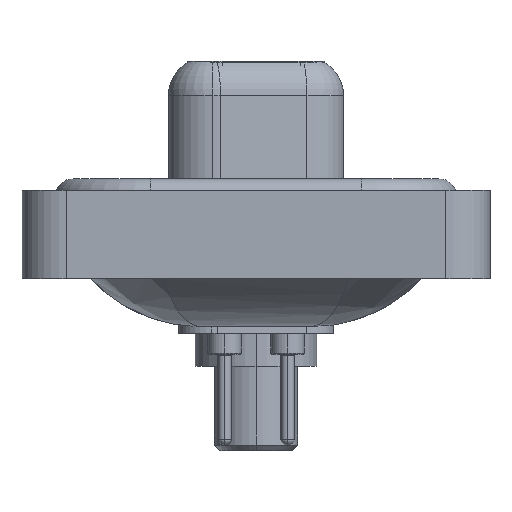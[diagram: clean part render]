
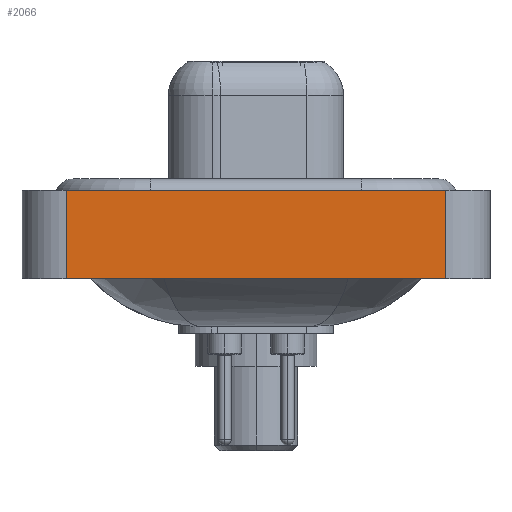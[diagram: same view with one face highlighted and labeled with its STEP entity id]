
A CAD part, left-side view. The second image highlights one B-rep face of the part: STEP entity #2066.
In plain terms, the highlighted planar face has unit normal (-1, 0, 0).
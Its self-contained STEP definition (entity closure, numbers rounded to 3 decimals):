
#321 = DIRECTION ( 'NONE',  ( 0., -1., 0. ) ) ;
#752 = LINE ( 'NONE', #3815, #19034 ) ;
#1023 = CARTESIAN_POINT ( 'NONE',  ( -7.25, -8.55, -3.6 ) ) ;
#1739 = ORIENTED_EDGE ( 'NONE', *, *, #3732, .F. ) ;
#2066 = ADVANCED_FACE ( 'NONE', ( #14321 ), #18576, .T. ) ;
#2612 = VECTOR ( 'NONE', #8266, 1000. ) ;
#2680 = VERTEX_POINT ( 'NONE', #13771 ) ;
#2856 = DIRECTION ( 'NONE',  ( 0., 0., 1. ) ) ;
#3732 = EDGE_CURVE ( 'NONE', #5099, #2680, #752, .T. ) ;
#3815 = CARTESIAN_POINT ( 'NONE',  ( -7.25, 8.55, -3.6 ) ) ;
#4140 = LINE ( 'NONE', #16198, #8108 ) ;
#4778 = VECTOR ( 'NONE', #321, 1000. ) ;
#4995 = ORIENTED_EDGE ( 'NONE', *, *, #15892, .T. ) ;
#5099 = VERTEX_POINT ( 'NONE', #9161 ) ;
#5203 = LINE ( 'NONE', #15603, #2612 ) ;
#6638 = EDGE_CURVE ( 'NONE', #2680, #16974, #8024, .T. ) ;
#6761 = DIRECTION ( 'NONE',  ( 0., 0., 1. ) ) ;
#6812 = ORIENTED_EDGE ( 'NONE', *, *, #9829, .T. ) ;
#8024 = LINE ( 'NONE', #17024, #4778 ) ;
#8108 = VECTOR ( 'NONE', #2856, 1000. ) ;
#8266 = DIRECTION ( 'NONE',  ( 0., -1., 0. ) ) ;
#9161 = CARTESIAN_POINT ( 'NONE',  ( -7.25, 8.55, -3.6 ) ) ;
#9829 = EDGE_CURVE ( 'NONE', #5099, #14279, #5203, .T. ) ;
#12650 = CARTESIAN_POINT ( 'NONE',  ( -7.25, -8.55, -3.6 ) ) ;
#13771 = CARTESIAN_POINT ( 'NONE',  ( -7.25, 8.55, 0.4 ) ) ;
#13804 = AXIS2_PLACEMENT_3D ( 'NONE', #12650, #14416, #18670 ) ;
#14279 = VERTEX_POINT ( 'NONE', #1023 ) ;
#14321 = FACE_OUTER_BOUND ( 'NONE', #16238, .T. ) ;
#14416 = DIRECTION ( 'NONE',  ( -1., 0., 0. ) ) ;
#15603 = CARTESIAN_POINT ( 'NONE',  ( -7.25, -8.55, -3.6 ) ) ;
#15892 = EDGE_CURVE ( 'NONE', #14279, #16974, #4140, .T. ) ;
#16198 = CARTESIAN_POINT ( 'NONE',  ( -7.25, -8.55, -3.6 ) ) ;
#16238 = EDGE_LOOP ( 'NONE', ( #4995, #18904, #1739, #6812 ) ) ;
#16623 = CARTESIAN_POINT ( 'NONE',  ( -7.25, -8.55, 0.4 ) ) ;
#16974 = VERTEX_POINT ( 'NONE', #16623 ) ;
#17024 = CARTESIAN_POINT ( 'NONE',  ( -7.25, -8.55, 0.4 ) ) ;
#18576 = PLANE ( 'NONE',  #13804 ) ;
#18670 = DIRECTION ( 'NONE',  ( 0., 0., 1. ) ) ;
#18904 = ORIENTED_EDGE ( 'NONE', *, *, #6638, .F. ) ;
#19034 = VECTOR ( 'NONE', #6761, 1000. ) ;
